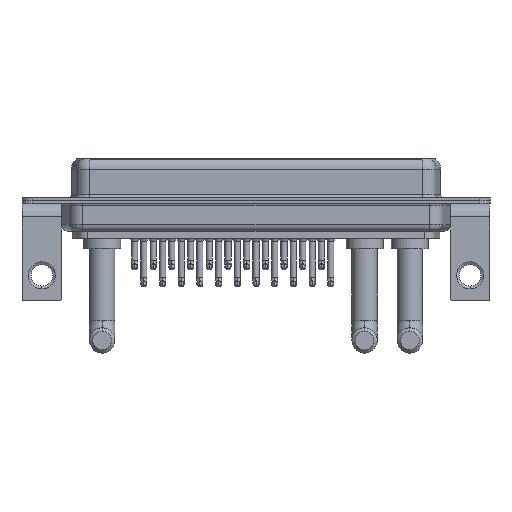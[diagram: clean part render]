
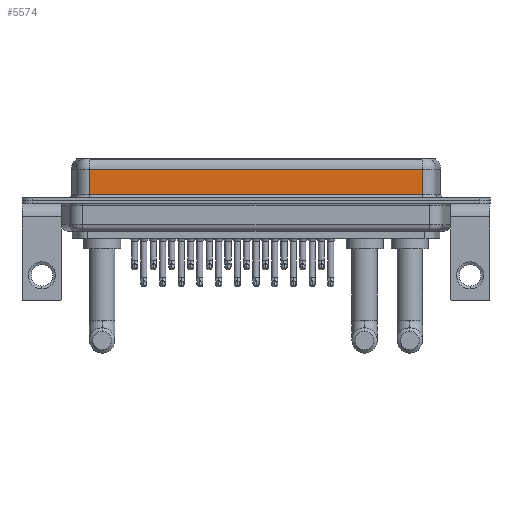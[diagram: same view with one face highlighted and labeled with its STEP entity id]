
A CAD part, front view. The second image highlights one B-rep face of the part: STEP entity #5574.
In plain terms, the highlighted planar face has unit normal (0, -1, 0).
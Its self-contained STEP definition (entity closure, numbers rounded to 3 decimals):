
#406 = CARTESIAN_POINT ( 'NONE',  ( 7.038, -3.95, 6.4 ) ) ;
#1208 = DIRECTION ( 'NONE',  ( 0., 1., 0. ) ) ;
#1334 = PLANE ( 'NONE',  #4928 ) ;
#1688 = DIRECTION ( 'NONE',  ( -1., 0., 0. ) ) ;
#2560 = CARTESIAN_POINT ( 'NONE',  ( 56.462, -3.95, 4.65 ) ) ;
#3388 = DIRECTION ( 'NONE',  ( 1., 0., 0. ) ) ;
#4120 = VECTOR ( 'NONE', #24057, 1000. ) ;
#4317 = FACE_OUTER_BOUND ( 'NONE', #9838, .T. ) ;
#4871 = LINE ( 'NONE', #12453, #4120 ) ;
#4928 = AXIS2_PLACEMENT_3D ( 'NONE', #8772, #1208, #8903 ) ;
#5574 = ADVANCED_FACE ( 'NONE', ( #4317 ), #1334, .F. ) ;
#6008 = VERTEX_POINT ( 'NONE', #2560 ) ;
#7436 = VECTOR ( 'NONE', #3388, 1000. ) ;
#8772 = CARTESIAN_POINT ( 'NONE',  ( 56.462, -3.95, 6.4 ) ) ;
#8903 = DIRECTION ( 'NONE',  ( 0., 0., 1. ) ) ;
#9838 = EDGE_LOOP ( 'NONE', ( #21618, #13677, #16855, #18098 ) ) ;
#10540 = VECTOR ( 'NONE', #1688, 1000. ) ;
#11126 = LINE ( 'NONE', #18724, #10540 ) ;
#11884 = CARTESIAN_POINT ( 'NONE',  ( 7.038, -3.95, 0.9 ) ) ;
#12069 = DIRECTION ( 'NONE',  ( 0., 0., -1. ) ) ;
#12393 = VERTEX_POINT ( 'NONE', #11884 ) ;
#12453 = CARTESIAN_POINT ( 'NONE',  ( 56.462, -3.95, 6.4 ) ) ;
#13677 = ORIENTED_EDGE ( 'NONE', *, *, #16738, .T. ) ;
#13868 = VERTEX_POINT ( 'NONE', #21058 ) ;
#15158 = VERTEX_POINT ( 'NONE', #24501 ) ;
#16738 = EDGE_CURVE ( 'NONE', #6008, #13868, #11126, .T. ) ;
#16855 = ORIENTED_EDGE ( 'NONE', *, *, #21775, .T. ) ;
#17436 = LINE ( 'NONE', #406, #23203 ) ;
#18098 = ORIENTED_EDGE ( 'NONE', *, *, #22550, .T. ) ;
#18724 = CARTESIAN_POINT ( 'NONE',  ( 56.462, -3.95, 4.65 ) ) ;
#20039 = LINE ( 'NONE', #20416, #7436 ) ;
#20171 = EDGE_CURVE ( 'NONE', #6008, #15158, #4871, .T. ) ;
#20416 = CARTESIAN_POINT ( 'NONE',  ( 56.462, -3.95, 0.9 ) ) ;
#21058 = CARTESIAN_POINT ( 'NONE',  ( 7.038, -3.95, 4.65 ) ) ;
#21618 = ORIENTED_EDGE ( 'NONE', *, *, #20171, .F. ) ;
#21775 = EDGE_CURVE ( 'NONE', #13868, #12393, #17436, .T. ) ;
#22550 = EDGE_CURVE ( 'NONE', #12393, #15158, #20039, .T. ) ;
#23203 = VECTOR ( 'NONE', #12069, 1000. ) ;
#24057 = DIRECTION ( 'NONE',  ( 0., 0., -1. ) ) ;
#24501 = CARTESIAN_POINT ( 'NONE',  ( 56.462, -3.95, 0.9 ) ) ;
